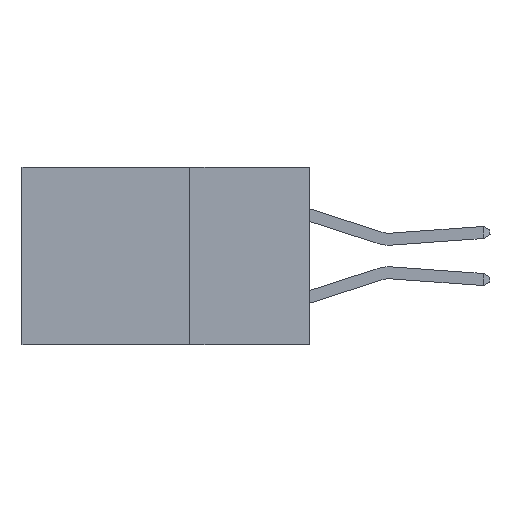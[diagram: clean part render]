
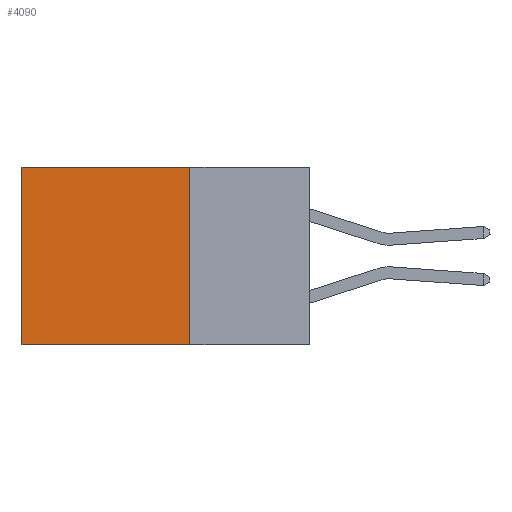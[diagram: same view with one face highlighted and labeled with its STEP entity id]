
A CAD part, left-side view. The second image highlights one B-rep face of the part: STEP entity #4090.
In plain terms, the highlighted planar face has unit normal (-1, 0, 0).
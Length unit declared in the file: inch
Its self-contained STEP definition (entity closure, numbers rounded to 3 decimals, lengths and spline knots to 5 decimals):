
#169 = VECTOR ( 'NONE', #16894, 39.37008 ) ;
#513 = VERTEX_POINT ( 'NONE', #4773 ) ;
#811 = VECTOR ( 'NONE', #19523, 39.37008 ) ;
#1178 = VERTEX_POINT ( 'NONE', #2771 ) ;
#1696 = CARTESIAN_POINT ( 'NONE',  ( 0.2615, 0.25, -0.37 ) ) ;
#2771 = CARTESIAN_POINT ( 'NONE',  ( 0.2615, 0.6, -0.37 ) ) ;
#3388 = FACE_OUTER_BOUND ( 'NONE', #14054, .T. ) ;
#3503 = DIRECTION ( 'NONE',  ( 1., 0., 0. ) ) ;
#3806 = DIRECTION ( 'NONE',  ( 0., 0., -1. ) ) ;
#4090 = ADVANCED_FACE ( 'NONE', ( #3388 ), #8774, .F. ) ;
#4536 = VERTEX_POINT ( 'NONE', #7372 ) ;
#4773 = CARTESIAN_POINT ( 'NONE',  ( 0.2615, 0.6, 0. ) ) ;
#5161 = AXIS2_PLACEMENT_3D ( 'NONE', #1696, #3503, #17419 ) ;
#6367 = CARTESIAN_POINT ( 'NONE',  ( 0.2615, 0.25, 0. ) ) ;
#7372 = CARTESIAN_POINT ( 'NONE',  ( 0.2615, 0.25, 0. ) ) ;
#7765 = CARTESIAN_POINT ( 'NONE',  ( 0.2615, 0.6, -0.37 ) ) ;
#7978 = ORIENTED_EDGE ( 'NONE', *, *, #11659, .T. ) ;
#8080 = LINE ( 'NONE', #7765, #811 ) ;
#8774 = PLANE ( 'NONE',  #5161 ) ;
#9031 = EDGE_CURVE ( 'NONE', #11604, #1178, #14875, .T. ) ;
#9960 = LINE ( 'NONE', #6367, #169 ) ;
#11604 = VERTEX_POINT ( 'NONE', #18271 ) ;
#11659 = EDGE_CURVE ( 'NONE', #513, #1178, #8080, .T. ) ;
#12307 = LINE ( 'NONE', #13979, #21260 ) ;
#12703 = VECTOR ( 'NONE', #12759, 39.37008 ) ;
#12759 = DIRECTION ( 'NONE',  ( 0., 1., 0. ) ) ;
#13979 = CARTESIAN_POINT ( 'NONE',  ( 0.2615, 0.25, -0.37 ) ) ;
#14054 = EDGE_LOOP ( 'NONE', ( #7978, #21945, #21991, #15596 ) ) ;
#14130 = EDGE_CURVE ( 'NONE', #4536, #513, #9960, .T. ) ;
#14875 = LINE ( 'NONE', #21718, #12703 ) ;
#15596 = ORIENTED_EDGE ( 'NONE', *, *, #14130, .T. ) ;
#16894 = DIRECTION ( 'NONE',  ( 0., 1., 0. ) ) ;
#17419 = DIRECTION ( 'NONE',  ( 0., 0., -1. ) ) ;
#18271 = CARTESIAN_POINT ( 'NONE',  ( 0.2615, 0.25, -0.37 ) ) ;
#19235 = EDGE_CURVE ( 'NONE', #4536, #11604, #12307, .T. ) ;
#19523 = DIRECTION ( 'NONE',  ( 0., 0., -1. ) ) ;
#21260 = VECTOR ( 'NONE', #3806, 39.37008 ) ;
#21718 = CARTESIAN_POINT ( 'NONE',  ( 0.2615, 0.25, -0.37 ) ) ;
#21945 = ORIENTED_EDGE ( 'NONE', *, *, #9031, .F. ) ;
#21991 = ORIENTED_EDGE ( 'NONE', *, *, #19235, .F. ) ;
